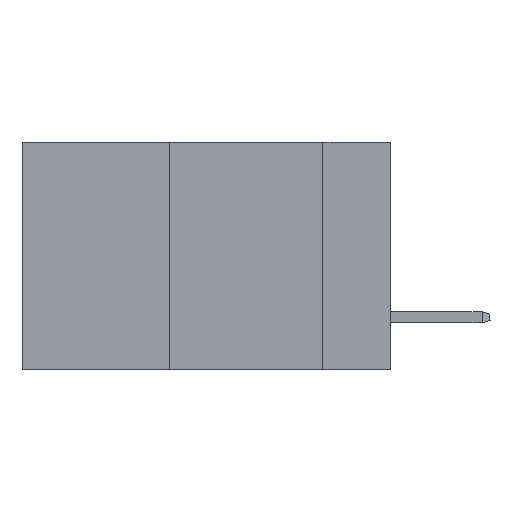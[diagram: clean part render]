
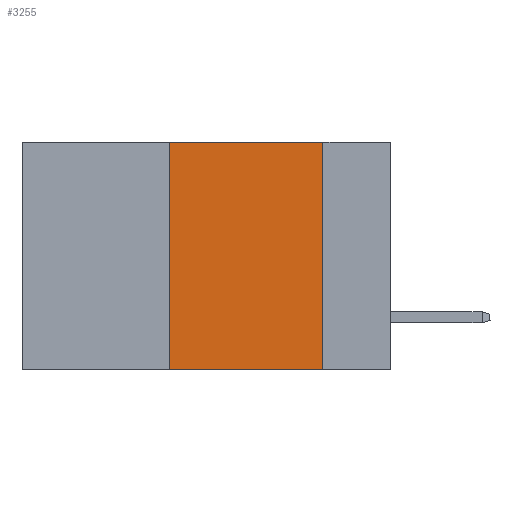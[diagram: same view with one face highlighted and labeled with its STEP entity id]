
A CAD part, left-side view. The second image highlights one B-rep face of the part: STEP entity #3255.
In plain terms, the highlighted planar face has unit normal (-1, 0, 0).
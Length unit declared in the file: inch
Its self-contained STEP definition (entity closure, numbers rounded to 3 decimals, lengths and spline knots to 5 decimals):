
#367 = VERTEX_POINT ( 'NONE', #2703 ) ;
#1797 = CARTESIAN_POINT ( 'NONE',  ( 0., 0.36, 0. ) ) ;
#2016 = VERTEX_POINT ( 'NONE', #11469 ) ;
#2092 = FACE_OUTER_BOUND ( 'NONE', #6309, .T. ) ;
#2485 = DIRECTION ( 'NONE',  ( 0., 0., -1. ) ) ;
#2701 = CARTESIAN_POINT ( 'NONE',  ( 0., 0.36, 0. ) ) ;
#2703 = CARTESIAN_POINT ( 'NONE',  ( 0., 0.11, 0. ) ) ;
#3255 = ADVANCED_FACE ( 'NONE', ( #2092 ), #14161, .F. ) ;
#3733 = DIRECTION ( 'NONE',  ( 0., 0., -1. ) ) ;
#4254 = DIRECTION ( 'NONE',  ( 0., -1., 0. ) ) ;
#4319 = ORIENTED_EDGE ( 'NONE', *, *, #14184, .T. ) ;
#4520 = VERTEX_POINT ( 'NONE', #1797 ) ;
#4889 = EDGE_CURVE ( 'NONE', #367, #8158, #7354, .T. ) ;
#5373 = CARTESIAN_POINT ( 'NONE',  ( 0., 0.6, -0.37 ) ) ;
#5824 = AXIS2_PLACEMENT_3D ( 'NONE', #8329, #9441, #2485 ) ;
#5901 = VECTOR ( 'NONE', #3733, 39.37008 ) ;
#6309 = EDGE_LOOP ( 'NONE', ( #9001, #7549, #11878, #4319 ) ) ;
#7354 = LINE ( 'NONE', #14299, #5901 ) ;
#7549 = ORIENTED_EDGE ( 'NONE', *, *, #10387, .F. ) ;
#7600 = VECTOR ( 'NONE', #12173, 39.37008 ) ;
#7764 = LINE ( 'NONE', #2701, #7600 ) ;
#7808 = DIRECTION ( 'NONE',  ( 0., -1., 0. ) ) ;
#8158 = VERTEX_POINT ( 'NONE', #14152 ) ;
#8329 = CARTESIAN_POINT ( 'NONE',  ( 0., 0.6, 0. ) ) ;
#8669 = EDGE_CURVE ( 'NONE', #2016, #4520, #7764, .T. ) ;
#9001 = ORIENTED_EDGE ( 'NONE', *, *, #4889, .F. ) ;
#9412 = VECTOR ( 'NONE', #4254, 39.37008 ) ;
#9441 = DIRECTION ( 'NONE',  ( 1., 0., 0. ) ) ;
#10387 = EDGE_CURVE ( 'NONE', #4520, #367, #11153, .T. ) ;
#11013 = VECTOR ( 'NONE', #7808, 39.37008 ) ;
#11153 = LINE ( 'NONE', #13468, #11013 ) ;
#11469 = CARTESIAN_POINT ( 'NONE',  ( 0., 0.36, -0.37 ) ) ;
#11878 = ORIENTED_EDGE ( 'NONE', *, *, #8669, .F. ) ;
#12173 = DIRECTION ( 'NONE',  ( 0., 0., 1. ) ) ;
#13468 = CARTESIAN_POINT ( 'NONE',  ( 0., 0.6, 0. ) ) ;
#14152 = CARTESIAN_POINT ( 'NONE',  ( 0., 0.11, -0.37 ) ) ;
#14161 = PLANE ( 'NONE',  #5824 ) ;
#14184 = EDGE_CURVE ( 'NONE', #2016, #8158, #14719, .T. ) ;
#14299 = CARTESIAN_POINT ( 'NONE',  ( 0., 0.11, 0. ) ) ;
#14719 = LINE ( 'NONE', #5373, #9412 ) ;
